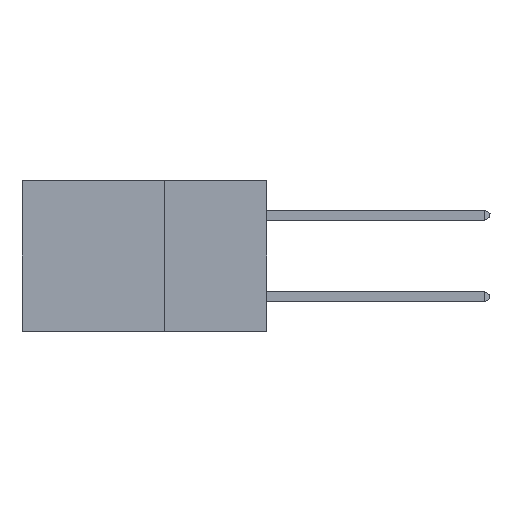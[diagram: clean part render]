
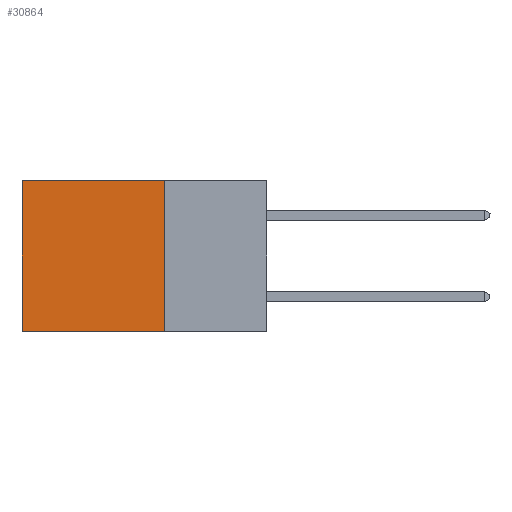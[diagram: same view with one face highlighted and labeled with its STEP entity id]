
A CAD part, left-side view. The second image highlights one B-rep face of the part: STEP entity #30864.
In plain terms, the highlighted planar face has unit normal (-1, 0, 0).
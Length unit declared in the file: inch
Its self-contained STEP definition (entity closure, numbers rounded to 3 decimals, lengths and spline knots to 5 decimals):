
#227 = EDGE_CURVE ( 'NONE', #3612, #29423, #12517, .T. ) ;
#682 = ORIENTED_EDGE ( 'NONE', *, *, #15150, .T. ) ;
#1477 = DIRECTION ( 'NONE',  ( 0., 0., -1. ) ) ;
#2387 = CARTESIAN_POINT ( 'NONE',  ( 0.2875, 0.6, 0. ) ) ;
#3612 = VERTEX_POINT ( 'NONE', #5584 ) ;
#4403 = VERTEX_POINT ( 'NONE', #20900 ) ;
#4436 = CARTESIAN_POINT ( 'NONE',  ( 0.2875, 0.25, 0. ) ) ;
#4469 = DIRECTION ( 'NONE',  ( 0., 1., 0. ) ) ;
#4934 = LINE ( 'NONE', #2387, #9954 ) ;
#5584 = CARTESIAN_POINT ( 'NONE',  ( 0.2875, 0.25, 0. ) ) ;
#7177 = LINE ( 'NONE', #13568, #9422 ) ;
#7279 = DIRECTION ( 'NONE',  ( 0., 1., 0. ) ) ;
#7386 = EDGE_LOOP ( 'NONE', ( #682, #21844, #32687, #25337 ) ) ;
#7962 = VERTEX_POINT ( 'NONE', #15214 ) ;
#8525 = EDGE_CURVE ( 'NONE', #3612, #7962, #29447, .T. ) ;
#9220 = PLANE ( 'NONE',  #10862 ) ;
#9422 = VECTOR ( 'NONE', #4469, 39.37008 ) ;
#9449 = EDGE_CURVE ( 'NONE', #29423, #4403, #7177, .T. ) ;
#9954 = VECTOR ( 'NONE', #21441, 39.37008 ) ;
#10862 = AXIS2_PLACEMENT_3D ( 'NONE', #11903, #22831, #1477 ) ;
#11282 = CARTESIAN_POINT ( 'NONE',  ( 0.2875, 0.25, -0.37 ) ) ;
#11903 = CARTESIAN_POINT ( 'NONE',  ( 0.2875, 0.25, 0. ) ) ;
#12517 = LINE ( 'NONE', #4436, #20792 ) ;
#13568 = CARTESIAN_POINT ( 'NONE',  ( 0.2875, 0.25, -0.37 ) ) ;
#15150 = EDGE_CURVE ( 'NONE', #7962, #4403, #4934, .T. ) ;
#15214 = CARTESIAN_POINT ( 'NONE',  ( 0.2875, 0.6, 0. ) ) ;
#15384 = DIRECTION ( 'NONE',  ( 0., 0., -1. ) ) ;
#15880 = CARTESIAN_POINT ( 'NONE',  ( 0.2875, 0.25, 0. ) ) ;
#20792 = VECTOR ( 'NONE', #15384, 39.37008 ) ;
#20900 = CARTESIAN_POINT ( 'NONE',  ( 0.2875, 0.6, -0.37 ) ) ;
#21441 = DIRECTION ( 'NONE',  ( 0., 0., -1. ) ) ;
#21844 = ORIENTED_EDGE ( 'NONE', *, *, #9449, .F. ) ;
#22831 = DIRECTION ( 'NONE',  ( 1., 0., 0. ) ) ;
#23547 = VECTOR ( 'NONE', #7279, 39.37008 ) ;
#25337 = ORIENTED_EDGE ( 'NONE', *, *, #8525, .T. ) ;
#26039 = FACE_OUTER_BOUND ( 'NONE', #7386, .T. ) ;
#29423 = VERTEX_POINT ( 'NONE', #11282 ) ;
#29447 = LINE ( 'NONE', #15880, #23547 ) ;
#30864 = ADVANCED_FACE ( 'NONE', ( #26039 ), #9220, .F. ) ;
#32687 = ORIENTED_EDGE ( 'NONE', *, *, #227, .F. ) ;
